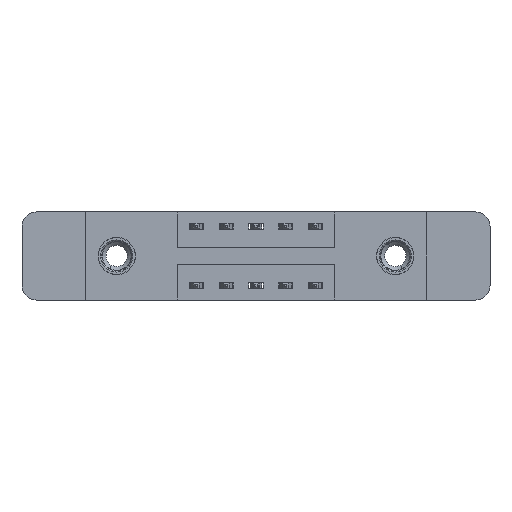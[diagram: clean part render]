
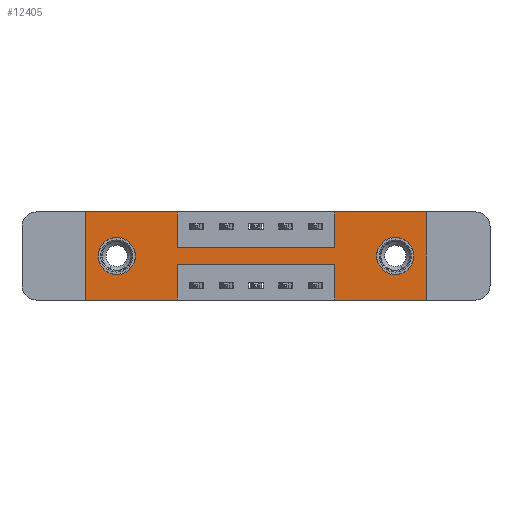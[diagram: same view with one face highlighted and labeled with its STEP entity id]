
A CAD part, front view. The second image highlights one B-rep face of the part: STEP entity #12405.
In plain terms, the highlighted planar face has unit normal (0, -1, 0).
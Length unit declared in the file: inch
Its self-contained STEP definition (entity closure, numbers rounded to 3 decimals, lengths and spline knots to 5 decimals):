
#37 = CARTESIAN_POINT ( 'NONE',  ( 0., 0., 0. ) ) ;
#82 = CARTESIAN_POINT ( 'NONE',  ( 1.3025, 0., -0.263 ) ) ;
#157 = EDGE_CURVE ( 'NONE', #12096, #13646, #5929, .T. ) ;
#200 = DIRECTION ( 'NONE',  ( 0., 0., 1. ) ) ;
#272 = CARTESIAN_POINT ( 'NONE',  ( 0., 0., 0. ) ) ;
#303 = VERTEX_POINT ( 'NONE', #2077 ) ;
#453 = DIRECTION ( 'NONE',  ( -1., 0., 0. ) ) ;
#455 = CARTESIAN_POINT ( 'NONE',  ( 0.1325, 0., -0.107 ) ) ;
#838 = VECTOR ( 'NONE', #4210, 39.37008 ) ;
#1045 = VECTOR ( 'NONE', #7639, 39.37008 ) ;
#1250 = VERTEX_POINT ( 'NONE', #13696 ) ;
#1388 = DIRECTION ( 'NONE',  ( 0., 0., -1. ) ) ;
#1461 = CARTESIAN_POINT ( 'NONE',  ( 0., 0., 0. ) ) ;
#1474 = EDGE_CURVE ( 'NONE', #13571, #12284, #12977, .T. ) ;
#1514 = CARTESIAN_POINT ( 'NONE',  ( 0., 0., -0.37 ) ) ;
#1527 = LINE ( 'NONE', #12320, #6839 ) ;
#1928 = EDGE_CURVE ( 'NONE', #10325, #1250, #4442, .T. ) ;
#2077 = CARTESIAN_POINT ( 'NONE',  ( 0.3875, 0., 0. ) ) ;
#2121 = CARTESIAN_POINT ( 'NONE',  ( 1.3025, 0., -0.107 ) ) ;
#2246 = CIRCLE ( 'NONE', #6712, 0.078 ) ;
#2327 = CARTESIAN_POINT ( 'NONE',  ( 0.3875, 0., -0.37 ) ) ;
#2351 = CARTESIAN_POINT ( 'NONE',  ( 0., 0., -0.37 ) ) ;
#2693 = ORIENTED_EDGE ( 'NONE', *, *, #4860, .F. ) ;
#2789 = FACE_OUTER_BOUND ( 'NONE', #6111, .T. ) ;
#2874 = CARTESIAN_POINT ( 'NONE',  ( 1.3025, 0., -0.185 ) ) ;
#2939 = EDGE_LOOP ( 'NONE', ( #6116, #3266 ) ) ;
#3103 = LINE ( 'NONE', #11514, #4660 ) ;
#3187 = VERTEX_POINT ( 'NONE', #6633 ) ;
#3261 = DIRECTION ( 'NONE',  ( -1., 0., 0. ) ) ;
#3266 = ORIENTED_EDGE ( 'NONE', *, *, #10144, .T. ) ;
#3354 = CIRCLE ( 'NONE', #7831, 0.078 ) ;
#3363 = AXIS2_PLACEMENT_3D ( 'NONE', #1514, #8028, #4727 ) ;
#3367 = CARTESIAN_POINT ( 'NONE',  ( 0.3875, 0., -0.15 ) ) ;
#3697 = CARTESIAN_POINT ( 'NONE',  ( 0.3875, 0., -0.15 ) ) ;
#3766 = ORIENTED_EDGE ( 'NONE', *, *, #6632, .F. ) ;
#3858 = ORIENTED_EDGE ( 'NONE', *, *, #10025, .F. ) ;
#3953 = EDGE_CURVE ( 'NONE', #1250, #12096, #6160, .T. ) ;
#4210 = DIRECTION ( 'NONE',  ( 1., 0., 0. ) ) ;
#4229 = DIRECTION ( 'NONE',  ( 0., 0., 1. ) ) ;
#4239 = ORIENTED_EDGE ( 'NONE', *, *, #3953, .F. ) ;
#4245 = CARTESIAN_POINT ( 'NONE',  ( 1.435, 0., -0.37 ) ) ;
#4442 = LINE ( 'NONE', #2351, #6353 ) ;
#4533 = ORIENTED_EDGE ( 'NONE', *, *, #1474, .F. ) ;
#4660 = VECTOR ( 'NONE', #6323, 39.37008 ) ;
#4709 = EDGE_CURVE ( 'NONE', #12520, #3187, #3103, .T. ) ;
#4727 = DIRECTION ( 'NONE',  ( 0., 0., -1. ) ) ;
#4860 = EDGE_CURVE ( 'NONE', #13646, #12520, #7570, .T. ) ;
#4884 = VERTEX_POINT ( 'NONE', #2121 ) ;
#5017 = EDGE_CURVE ( 'NONE', #4884, #11833, #13655, .T. ) ;
#5283 = CARTESIAN_POINT ( 'NONE',  ( 0.3875, 0., -0.37 ) ) ;
#5617 = LINE ( 'NONE', #272, #10664 ) ;
#5650 = VERTEX_POINT ( 'NONE', #10673 ) ;
#5657 = CARTESIAN_POINT ( 'NONE',  ( 0.1325, 0., -0.185 ) ) ;
#5723 = DIRECTION ( 'NONE',  ( 0., 0., 1. ) ) ;
#5807 = DIRECTION ( 'NONE',  ( 0., 0., -1. ) ) ;
#5884 = DIRECTION ( 'NONE',  ( 0., 1., 0. ) ) ;
#5929 = LINE ( 'NONE', #8931, #12710 ) ;
#5987 = EDGE_CURVE ( 'NONE', #5650, #6551, #3354, .T. ) ;
#6111 = EDGE_LOOP ( 'NONE', ( #2693, #6756, #4239, #6447, #10514, #8121, #3766, #4533, #6787, #3858, #11285, #7358 ) ) ;
#6116 = ORIENTED_EDGE ( 'NONE', *, *, #5017, .T. ) ;
#6160 = LINE ( 'NONE', #12399, #12409 ) ;
#6249 = VECTOR ( 'NONE', #5723, 39.37008 ) ;
#6323 = DIRECTION ( 'NONE',  ( -1., 0., 0. ) ) ;
#6353 = VECTOR ( 'NONE', #3261, 39.37008 ) ;
#6447 = ORIENTED_EDGE ( 'NONE', *, *, #1928, .F. ) ;
#6551 = VERTEX_POINT ( 'NONE', #455 ) ;
#6632 = EDGE_CURVE ( 'NONE', #12284, #13250, #12170, .T. ) ;
#6633 = CARTESIAN_POINT ( 'NONE',  ( 0., 0., -0.37 ) ) ;
#6692 = VECTOR ( 'NONE', #4229, 39.37008 ) ;
#6707 = CARTESIAN_POINT ( 'NONE',  ( 1.0475, 0., -0.22 ) ) ;
#6712 = AXIS2_PLACEMENT_3D ( 'NONE', #5657, #13162, #9998 ) ;
#6756 = ORIENTED_EDGE ( 'NONE', *, *, #157, .F. ) ;
#6787 = ORIENTED_EDGE ( 'NONE', *, *, #7996, .F. ) ;
#6836 = CARTESIAN_POINT ( 'NONE',  ( 1.0475, 0., 0. ) ) ;
#6839 = VECTOR ( 'NONE', #5807, 39.37008 ) ;
#6849 = VERTEX_POINT ( 'NONE', #10677 ) ;
#6885 = EDGE_CURVE ( 'NONE', #3187, #7111, #9639, .T. ) ;
#7030 = PLANE ( 'NONE',  #3363 ) ;
#7065 = DIRECTION ( 'NONE',  ( 0., 0., -1. ) ) ;
#7111 = VERTEX_POINT ( 'NONE', #11521 ) ;
#7336 = CARTESIAN_POINT ( 'NONE',  ( 1.3025, 0., -0.185 ) ) ;
#7358 = ORIENTED_EDGE ( 'NONE', *, *, #4709, .F. ) ;
#7470 = EDGE_CURVE ( 'NONE', #13250, #6849, #5617, .T. ) ;
#7570 = LINE ( 'NONE', #2327, #11615 ) ;
#7639 = DIRECTION ( 'NONE',  ( 1., 0., 0. ) ) ;
#7779 = ORIENTED_EDGE ( 'NONE', *, *, #12142, .T. ) ;
#7815 = AXIS2_PLACEMENT_3D ( 'NONE', #7336, #10574, #7065 ) ;
#7831 = AXIS2_PLACEMENT_3D ( 'NONE', #13496, #9191, #200 ) ;
#7985 = CARTESIAN_POINT ( 'NONE',  ( 0.3875, 0., -0.22 ) ) ;
#7996 = EDGE_CURVE ( 'NONE', #303, #13571, #1527, .T. ) ;
#8028 = DIRECTION ( 'NONE',  ( 0., -1., 0. ) ) ;
#8100 = FACE_BOUND ( 'NONE', #2939, .T. ) ;
#8121 = ORIENTED_EDGE ( 'NONE', *, *, #7470, .F. ) ;
#8267 = ORIENTED_EDGE ( 'NONE', *, *, #5987, .T. ) ;
#8269 = VECTOR ( 'NONE', #1388, 39.37008 ) ;
#8931 = CARTESIAN_POINT ( 'NONE',  ( 0.3875, 0., -0.22 ) ) ;
#9191 = DIRECTION ( 'NONE',  ( 0., 1., 0. ) ) ;
#9334 = AXIS2_PLACEMENT_3D ( 'NONE', #2874, #5884, #12391 ) ;
#9639 = LINE ( 'NONE', #37, #6692 ) ;
#9998 = DIRECTION ( 'NONE',  ( 0., 0., 1. ) ) ;
#10025 = EDGE_CURVE ( 'NONE', #7111, #303, #10087, .T. ) ;
#10087 = LINE ( 'NONE', #1461, #838 ) ;
#10144 = EDGE_CURVE ( 'NONE', #11833, #4884, #10690, .T. ) ;
#10325 = VERTEX_POINT ( 'NONE', #4245 ) ;
#10514 = ORIENTED_EDGE ( 'NONE', *, *, #12098, .F. ) ;
#10574 = DIRECTION ( 'NONE',  ( 0., 1., 0. ) ) ;
#10664 = VECTOR ( 'NONE', #13542, 39.37008 ) ;
#10673 = CARTESIAN_POINT ( 'NONE',  ( 0.1325, 0., -0.263 ) ) ;
#10677 = CARTESIAN_POINT ( 'NONE',  ( 1.435, 0., 0. ) ) ;
#10690 = CIRCLE ( 'NONE', #9334, 0.078 ) ;
#10767 = CARTESIAN_POINT ( 'NONE',  ( 1.435, 0., 0. ) ) ;
#11285 = ORIENTED_EDGE ( 'NONE', *, *, #6885, .F. ) ;
#11426 = DIRECTION ( 'NONE',  ( 0., 0., 1. ) ) ;
#11514 = CARTESIAN_POINT ( 'NONE',  ( 0., 0., -0.37 ) ) ;
#11521 = CARTESIAN_POINT ( 'NONE',  ( 0., 0., 0. ) ) ;
#11615 = VECTOR ( 'NONE', #11719, 39.37008 ) ;
#11719 = DIRECTION ( 'NONE',  ( 0., 0., -1. ) ) ;
#11833 = VERTEX_POINT ( 'NONE', #82 ) ;
#11968 = LINE ( 'NONE', #10767, #8269 ) ;
#12096 = VERTEX_POINT ( 'NONE', #6707 ) ;
#12098 = EDGE_CURVE ( 'NONE', #6849, #10325, #11968, .T. ) ;
#12142 = EDGE_CURVE ( 'NONE', #6551, #5650, #2246, .T. ) ;
#12169 = CARTESIAN_POINT ( 'NONE',  ( 1.0475, 0., -0.15 ) ) ;
#12170 = LINE ( 'NONE', #6836, #6249 ) ;
#12284 = VERTEX_POINT ( 'NONE', #12169 ) ;
#12320 = CARTESIAN_POINT ( 'NONE',  ( 0.3875, 0., 0. ) ) ;
#12371 = FACE_BOUND ( 'NONE', #13333, .T. ) ;
#12391 = DIRECTION ( 'NONE',  ( 0., 0., -1. ) ) ;
#12399 = CARTESIAN_POINT ( 'NONE',  ( 1.0475, 0., -0.37 ) ) ;
#12405 = ADVANCED_FACE ( 'NONE', ( #8100, #12371, #2789 ), #7030, .T. ) ;
#12409 = VECTOR ( 'NONE', #11426, 39.37008 ) ;
#12520 = VERTEX_POINT ( 'NONE', #5283 ) ;
#12710 = VECTOR ( 'NONE', #453, 39.37008 ) ;
#12977 = LINE ( 'NONE', #3367, #1045 ) ;
#13162 = DIRECTION ( 'NONE',  ( 0., 1., 0. ) ) ;
#13199 = CARTESIAN_POINT ( 'NONE',  ( 1.0475, 0., 0. ) ) ;
#13250 = VERTEX_POINT ( 'NONE', #13199 ) ;
#13333 = EDGE_LOOP ( 'NONE', ( #7779, #8267 ) ) ;
#13496 = CARTESIAN_POINT ( 'NONE',  ( 0.1325, 0., -0.185 ) ) ;
#13542 = DIRECTION ( 'NONE',  ( 1., 0., 0. ) ) ;
#13571 = VERTEX_POINT ( 'NONE', #3697 ) ;
#13646 = VERTEX_POINT ( 'NONE', #7985 ) ;
#13655 = CIRCLE ( 'NONE', #7815, 0.078 ) ;
#13696 = CARTESIAN_POINT ( 'NONE',  ( 1.0475, 0., -0.37 ) ) ;
